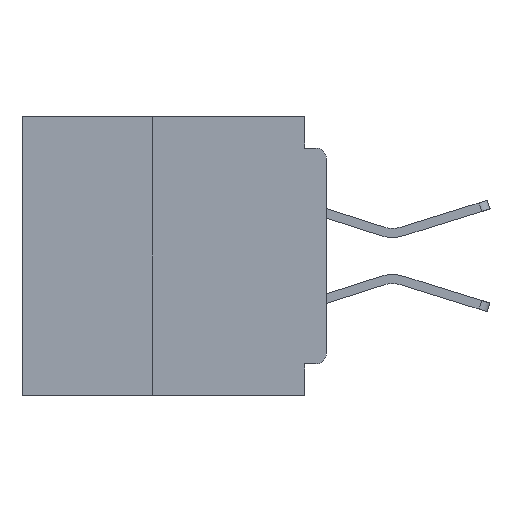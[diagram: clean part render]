
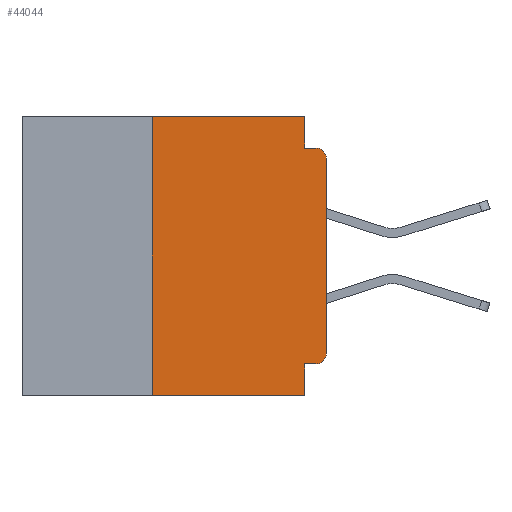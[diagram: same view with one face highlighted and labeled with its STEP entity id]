
A CAD part, left-side view. The second image highlights one B-rep face of the part: STEP entity #44044.
In plain terms, the highlighted planar face has unit normal (-1, 0, 0).
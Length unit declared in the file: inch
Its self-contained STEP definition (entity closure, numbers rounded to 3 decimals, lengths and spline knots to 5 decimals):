
#552 = ORIENTED_EDGE ( 'NONE', *, *, #34307, .T. ) ;
#1186 = VECTOR ( 'NONE', #5377, 39.37008 ) ;
#2080 = ORIENTED_EDGE ( 'NONE', *, *, #59617, .F. ) ;
#2643 = LINE ( 'NONE', #42142, #1186 ) ;
#2709 = ORIENTED_EDGE ( 'NONE', *, *, #46704, .F. ) ;
#2744 = DIRECTION ( 'NONE',  ( 0., 0., -1. ) ) ;
#3125 = DIRECTION ( 'NONE',  ( 0., 0., 1. ) ) ;
#3285 = CARTESIAN_POINT ( 'NONE',  ( 0., 0.437, 0. ) ) ;
#3609 = FACE_OUTER_BOUND ( 'NONE', #44865, .T. ) ;
#3961 = VERTEX_POINT ( 'NONE', #42624 ) ;
#4284 = AXIS2_PLACEMENT_3D ( 'NONE', #21550, #53585, #26146 ) ;
#4536 = VERTEX_POINT ( 'NONE', #56044 ) ;
#4799 = CARTESIAN_POINT ( 'NONE',  ( 0., 0.031, -0.355 ) ) ;
#5061 = ORIENTED_EDGE ( 'NONE', *, *, #44216, .F. ) ;
#5377 = DIRECTION ( 'NONE',  ( 0., -1., 0. ) ) ;
#5401 = EDGE_CURVE ( 'NONE', #27605, #10555, #52855, .T. ) ;
#5567 = LINE ( 'NONE', #43392, #28630 ) ;
#5783 = VECTOR ( 'NONE', #46091, 39.37008 ) ;
#6437 = VERTEX_POINT ( 'NONE', #25136 ) ;
#7196 = LINE ( 'NONE', #7704, #43846 ) ;
#7704 = CARTESIAN_POINT ( 'NONE',  ( 0., 0.031, 0. ) ) ;
#7944 = DIRECTION ( 'NONE',  ( 0., 0., -1. ) ) ;
#8866 = CARTESIAN_POINT ( 'NONE',  ( 0., 0.437, -0.4 ) ) ;
#10555 = VERTEX_POINT ( 'NONE', #4799 ) ;
#11705 = ORIENTED_EDGE ( 'NONE', *, *, #5401, .F. ) ;
#11970 = AXIS2_PLACEMENT_3D ( 'NONE', #57862, #30356, #2744 ) ;
#12320 = ORIENTED_EDGE ( 'NONE', *, *, #49352, .F. ) ;
#12541 = VECTOR ( 'NONE', #3125, 39.37008 ) ;
#15876 = VERTEX_POINT ( 'NONE', #47268 ) ;
#16264 = CARTESIAN_POINT ( 'NONE',  ( 0., 0.031, -0.4 ) ) ;
#16274 = VECTOR ( 'NONE', #17221, 39.37008 ) ;
#17221 = DIRECTION ( 'NONE',  ( 0., 1., 0. ) ) ;
#19227 = VERTEX_POINT ( 'NONE', #16264 ) ;
#19565 = LINE ( 'NONE', #41482, #5783 ) ;
#20216 = CARTESIAN_POINT ( 'NONE',  ( 0., 0., -0.34 ) ) ;
#20600 = EDGE_CURVE ( 'NONE', #48857, #3961, #27680, .T. ) ;
#21550 = CARTESIAN_POINT ( 'NONE',  ( 0., 0.015, -0.06 ) ) ;
#22240 = CARTESIAN_POINT ( 'NONE',  ( 0., 0., -0.355 ) ) ;
#22807 = DIRECTION ( 'NONE',  ( 0., -1., 0. ) ) ;
#23310 = ORIENTED_EDGE ( 'NONE', *, *, #20600, .T. ) ;
#24899 = CIRCLE ( 'NONE', #11970, 0.015 ) ;
#25136 = CARTESIAN_POINT ( 'NONE',  ( 0., 0.031, 0. ) ) ;
#26146 = DIRECTION ( 'NONE',  ( 0., 0., -1. ) ) ;
#27133 = CARTESIAN_POINT ( 'NONE',  ( 0., 0.031, -0.4 ) ) ;
#27605 = VERTEX_POINT ( 'NONE', #34356 ) ;
#27680 = LINE ( 'NONE', #30723, #12541 ) ;
#28376 = ORIENTED_EDGE ( 'NONE', *, *, #55866, .T. ) ;
#28630 = VECTOR ( 'NONE', #48021, 39.37008 ) ;
#30356 = DIRECTION ( 'NONE',  ( -1., 0., 0. ) ) ;
#30435 = VECTOR ( 'NONE', #31690, 39.37008 ) ;
#30723 = CARTESIAN_POINT ( 'NONE',  ( 0., 0., 0. ) ) ;
#31690 = DIRECTION ( 'NONE',  ( 0., 0., -1. ) ) ;
#32103 = LINE ( 'NONE', #8866, #42850 ) ;
#34307 = EDGE_CURVE ( 'NONE', #27605, #48857, #24899, .T. ) ;
#34356 = CARTESIAN_POINT ( 'NONE',  ( 0., 0.015, -0.355 ) ) ;
#34803 = ORIENTED_EDGE ( 'NONE', *, *, #41144, .T. ) ;
#34997 = EDGE_CURVE ( 'NONE', #10555, #19227, #43277, .T. ) ;
#35497 = DIRECTION ( 'NONE',  ( 1., 0., 0. ) ) ;
#41144 = EDGE_CURVE ( 'NONE', #50765, #19227, #32103, .T. ) ;
#41482 = CARTESIAN_POINT ( 'NONE',  ( 0., 0.25, -0.4 ) ) ;
#42142 = CARTESIAN_POINT ( 'NONE',  ( 0., 0., -0.045 ) ) ;
#42624 = CARTESIAN_POINT ( 'NONE',  ( 0., 0., -0.06 ) ) ;
#42850 = VECTOR ( 'NONE', #22807, 39.37008 ) ;
#43277 = LINE ( 'NONE', #27133, #30435 ) ;
#43392 = CARTESIAN_POINT ( 'NONE',  ( 0., 0.437, 0. ) ) ;
#43846 = VECTOR ( 'NONE', #44448, 39.37008 ) ;
#44044 = ADVANCED_FACE ( 'NONE', ( #3609 ), #44502, .F. ) ;
#44216 = EDGE_CURVE ( 'NONE', #50765, #15876, #19565, .T. ) ;
#44448 = DIRECTION ( 'NONE',  ( 0., 0., -1. ) ) ;
#44502 = PLANE ( 'NONE',  #53516 ) ;
#44865 = EDGE_LOOP ( 'NONE', ( #23310, #28376, #12320, #2080, #2709, #5061, #34803, #56333, #11705, #552 ) ) ;
#46091 = DIRECTION ( 'NONE',  ( 0., 0., 1. ) ) ;
#46704 = EDGE_CURVE ( 'NONE', #15876, #6437, #5567, .T. ) ;
#47268 = CARTESIAN_POINT ( 'NONE',  ( 0., 0.25, 0. ) ) ;
#48021 = DIRECTION ( 'NONE',  ( 0., -1., 0. ) ) ;
#48857 = VERTEX_POINT ( 'NONE', #20216 ) ;
#49352 = EDGE_CURVE ( 'NONE', #4536, #53791, #2643, .T. ) ;
#50321 = CARTESIAN_POINT ( 'NONE',  ( 0., 0.015, -0.045 ) ) ;
#50765 = VERTEX_POINT ( 'NONE', #52233 ) ;
#52233 = CARTESIAN_POINT ( 'NONE',  ( 0., 0.25, -0.4 ) ) ;
#52855 = LINE ( 'NONE', #22240, #16274 ) ;
#53516 = AXIS2_PLACEMENT_3D ( 'NONE', #3285, #35497, #7944 ) ;
#53585 = DIRECTION ( 'NONE',  ( -1., 0., 0. ) ) ;
#53791 = VERTEX_POINT ( 'NONE', #50321 ) ;
#55866 = EDGE_CURVE ( 'NONE', #3961, #53791, #57237, .T. ) ;
#56044 = CARTESIAN_POINT ( 'NONE',  ( 0., 0.031, -0.045 ) ) ;
#56333 = ORIENTED_EDGE ( 'NONE', *, *, #34997, .F. ) ;
#57237 = CIRCLE ( 'NONE', #4284, 0.015 ) ;
#57862 = CARTESIAN_POINT ( 'NONE',  ( 0., 0.015, -0.34 ) ) ;
#59617 = EDGE_CURVE ( 'NONE', #6437, #4536, #7196, .T. ) ;
